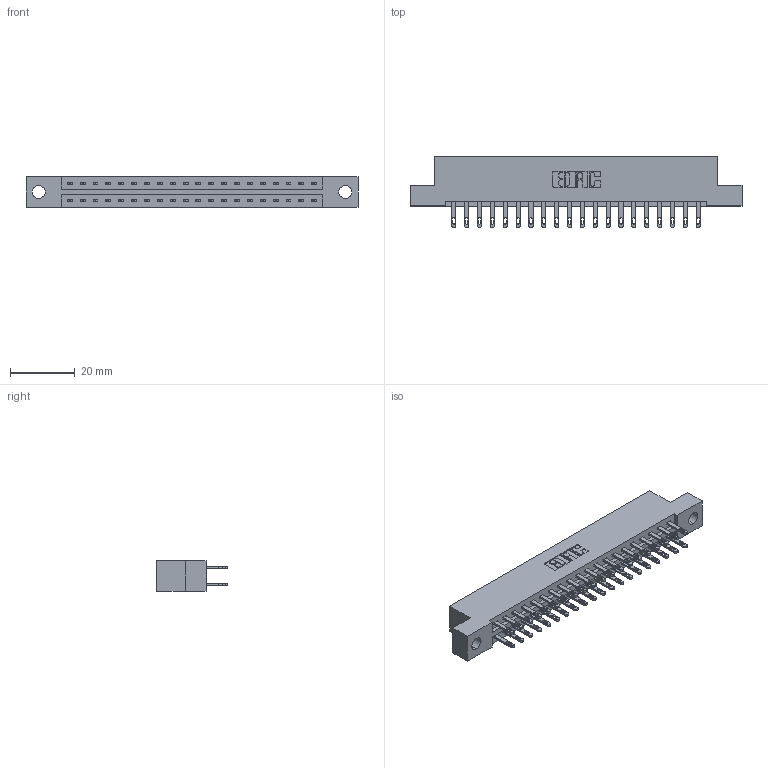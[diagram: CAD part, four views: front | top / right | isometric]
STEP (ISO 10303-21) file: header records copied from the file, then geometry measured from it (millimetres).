
FILE_DESCRIPTION (( 'STEP AP203' ), '1' );
FILE_NAME ('337-040-500-204.STEP', '2019-10-09T11:15:22', ( '' ), ( '' ), 'SwSTEP 2.0', 'SolidWorks 2016', '' );
FILE_SCHEMA (( 'CONFIG_CONTROL_DESIGN' ));
Length unit declared in the file: inch
Products named in the file (3): 337-040-500-204; 345-292-001_345-293-100; 337 Part_Flush Mounting Lugs - 0.156 Dia-TH
Assembly tree (41 placements, depth 2):
  337-040-500-204
    337 Part_Flush Mounting Lugs - 0.156 Dia-TH
    345-292-001_345-293-100  x40
Bounding box: 102.26 x 21.85 x 9.4 mm (x, y, z)
Volume: 10518.5 mm3; surface area: 11918.8 mm2
Topology: 41 solids, 41 shells, 2114 faces, 6431 edges, 4286 vertices
Faces by surface type: plane 1350, cylinder 764
Entity records: 18285 total; most frequent: CARTESIAN_POINT 3098, ORIENTED_EDGE 3034, DIRECTION 2677, EDGE_CURVE 1517, VECTOR 1385, LINE 1385, VERTEX_POINT 1010, AXIS2_PLACEMENT_3D 646
